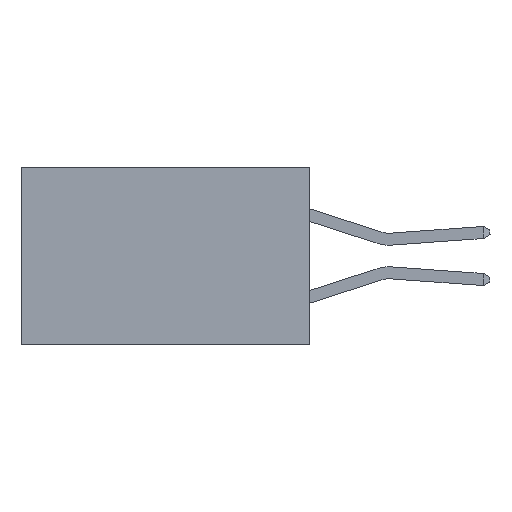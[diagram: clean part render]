
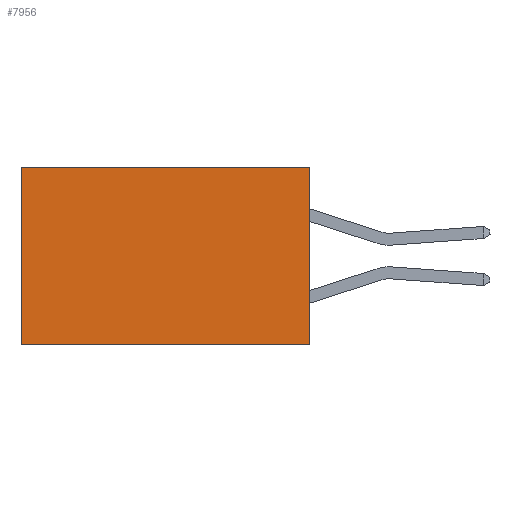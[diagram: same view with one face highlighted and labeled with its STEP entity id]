
A CAD part, left-side view. The second image highlights one B-rep face of the part: STEP entity #7956.
In plain terms, the highlighted planar face has unit normal (-1, 0, 0).
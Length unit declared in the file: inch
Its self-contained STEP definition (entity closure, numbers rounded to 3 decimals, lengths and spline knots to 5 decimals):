
#635 = DIRECTION ( 'NONE',  ( 0., 0., -1. ) ) ;
#931 = ORIENTED_EDGE ( 'NONE', *, *, #20389, .T. ) ;
#2253 = LINE ( 'NONE', #7887, #8650 ) ;
#4168 = FACE_OUTER_BOUND ( 'NONE', #19222, .T. ) ;
#4216 = CARTESIAN_POINT ( 'NONE',  ( 0.298, 0., 0. ) ) ;
#4308 = CARTESIAN_POINT ( 'NONE',  ( 0.298, 0., 0. ) ) ;
#4537 = EDGE_CURVE ( 'NONE', #8841, #9795, #2253, .T. ) ;
#4569 = DIRECTION ( 'NONE',  ( 0., 1., 0. ) ) ;
#4675 = CARTESIAN_POINT ( 'NONE',  ( 0.298, 0., 0. ) ) ;
#4985 = AXIS2_PLACEMENT_3D ( 'NONE', #4675, #12808, #635 ) ;
#5039 = CARTESIAN_POINT ( 'NONE',  ( 0.298, 0.6, 0. ) ) ;
#5555 = VECTOR ( 'NONE', #4569, 39.37008 ) ;
#6731 = VERTEX_POINT ( 'NONE', #4216 ) ;
#7887 = CARTESIAN_POINT ( 'NONE',  ( 0.298, 0., -0.37 ) ) ;
#7956 = ADVANCED_FACE ( 'NONE', ( #4168 ), #10787, .F. ) ;
#8189 = CARTESIAN_POINT ( 'NONE',  ( 0.298, 0.6, -0.37 ) ) ;
#8650 = VECTOR ( 'NONE', #18361, 39.37008 ) ;
#8841 = VERTEX_POINT ( 'NONE', #13388 ) ;
#9289 = ORIENTED_EDGE ( 'NONE', *, *, #14509, .F. ) ;
#9795 = VERTEX_POINT ( 'NONE', #8189 ) ;
#10787 = PLANE ( 'NONE',  #4985 ) ;
#11563 = LINE ( 'NONE', #18653, #5555 ) ;
#12447 = DIRECTION ( 'NONE',  ( 0., 0., -1. ) ) ;
#12752 = EDGE_CURVE ( 'NONE', #6731, #25220, #11563, .T. ) ;
#12808 = DIRECTION ( 'NONE',  ( 1., 0., 0. ) ) ;
#13388 = CARTESIAN_POINT ( 'NONE',  ( 0.298, 0., -0.37 ) ) ;
#13416 = VECTOR ( 'NONE', #12447, 39.37008 ) ;
#13465 = LINE ( 'NONE', #15368, #18161 ) ;
#14509 = EDGE_CURVE ( 'NONE', #6731, #8841, #23964, .T. ) ;
#15368 = CARTESIAN_POINT ( 'NONE',  ( 0.298, 0.6, 0. ) ) ;
#15984 = ORIENTED_EDGE ( 'NONE', *, *, #4537, .F. ) ;
#17368 = DIRECTION ( 'NONE',  ( 0., 0., -1. ) ) ;
#18161 = VECTOR ( 'NONE', #17368, 39.37008 ) ;
#18361 = DIRECTION ( 'NONE',  ( 0., 1., 0. ) ) ;
#18653 = CARTESIAN_POINT ( 'NONE',  ( 0.298, 0., 0. ) ) ;
#19222 = EDGE_LOOP ( 'NONE', ( #931, #15984, #9289, #20902 ) ) ;
#20389 = EDGE_CURVE ( 'NONE', #25220, #9795, #13465, .T. ) ;
#20902 = ORIENTED_EDGE ( 'NONE', *, *, #12752, .T. ) ;
#23964 = LINE ( 'NONE', #4308, #13416 ) ;
#25220 = VERTEX_POINT ( 'NONE', #5039 ) ;
